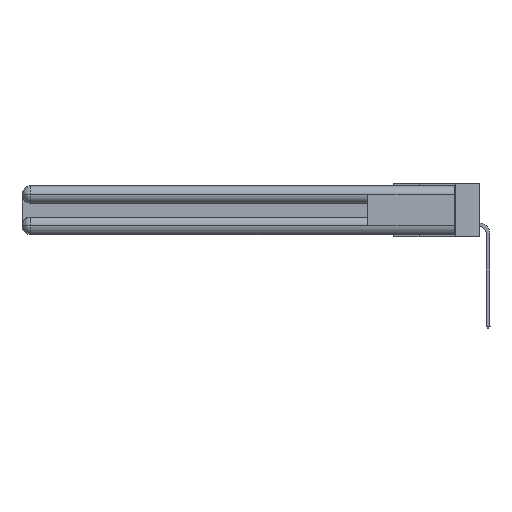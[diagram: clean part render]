
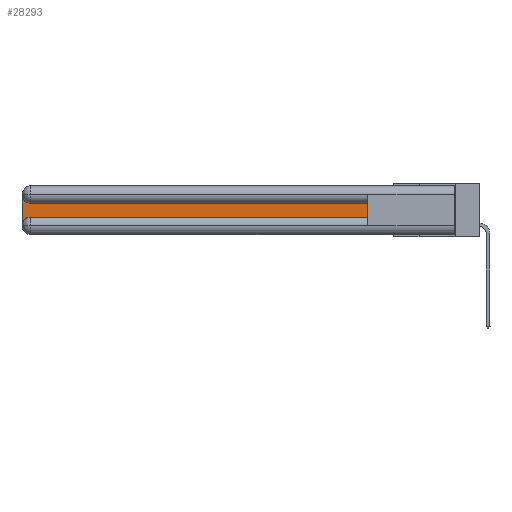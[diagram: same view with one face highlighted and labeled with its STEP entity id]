
A CAD part, left-side view. The second image highlights one B-rep face of the part: STEP entity #28293.
In plain terms, the highlighted planar face has unit normal (-1, 0, 0).
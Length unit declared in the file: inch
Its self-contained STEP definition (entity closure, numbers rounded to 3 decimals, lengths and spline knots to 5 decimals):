
#771 = VERTEX_POINT ( 'NONE', #12176 ) ;
#1724 = LINE ( 'NONE', #11737, #24600 ) ;
#2594 = ORIENTED_EDGE ( 'NONE', *, *, #15719, .T. ) ;
#4088 = DIRECTION ( 'NONE',  ( 1., 0., 0. ) ) ;
#4320 = CARTESIAN_POINT ( 'NONE',  ( 0.075, 3., -0.0625 ) ) ;
#4334 = VECTOR ( 'NONE', #18008, 39.37008 ) ;
#4375 = PLANE ( 'NONE',  #28291 ) ;
#5604 = VERTEX_POINT ( 'NONE', #19478 ) ;
#6372 = DIRECTION ( 'NONE',  ( 0., 0., -1. ) ) ;
#8468 = EDGE_CURVE ( 'NONE', #12946, #21386, #15218, .T. ) ;
#8684 = FACE_OUTER_BOUND ( 'NONE', #12983, .T. ) ;
#8936 = CARTESIAN_POINT ( 'NONE',  ( 0.075, 0.6, -0.1225 ) ) ;
#9541 = CARTESIAN_POINT ( 'NONE',  ( 0.075, 3., -0.1225 ) ) ;
#10247 = CARTESIAN_POINT ( 'NONE',  ( 0.075, 0.6, -0.2175 ) ) ;
#10462 = EDGE_CURVE ( 'NONE', #17507, #771, #27649, .T. ) ;
#11031 = CARTESIAN_POINT ( 'NONE',  ( 0.075, 2.94, -0.0625 ) ) ;
#11171 = ORIENTED_EDGE ( 'NONE', *, *, #8468, .T. ) ;
#11715 = CIRCLE ( 'NONE', #22199, 0.06 ) ;
#11737 = CARTESIAN_POINT ( 'NONE',  ( 0.075, 0.6, -0.2175 ) ) ;
#12176 = CARTESIAN_POINT ( 'NONE',  ( 0.075, 0.6, -0.2175 ) ) ;
#12946 = VERTEX_POINT ( 'NONE', #4320 ) ;
#12983 = EDGE_LOOP ( 'NONE', ( #19343, #2594, #11171, #23024, #16053, #21503 ) ) ;
#14130 = DIRECTION ( 'NONE',  ( 0., 0., 1. ) ) ;
#14459 = CARTESIAN_POINT ( 'NONE',  ( 0.075, 2.94, -0.2175 ) ) ;
#15218 = LINE ( 'NONE', #20277, #4334 ) ;
#15719 = EDGE_CURVE ( 'NONE', #5604, #12946, #28350, .T. ) ;
#16053 = ORIENTED_EDGE ( 'NONE', *, *, #10462, .T. ) ;
#16295 = EDGE_CURVE ( 'NONE', #771, #18937, #1724, .T. ) ;
#16494 = DIRECTION ( 'NONE',  ( 0., 1., 0. ) ) ;
#16663 = DIRECTION ( 'NONE',  ( 1., 0., 0. ) ) ;
#16953 = CARTESIAN_POINT ( 'NONE',  ( 0.075, 3., -0.2775 ) ) ;
#17507 = VERTEX_POINT ( 'NONE', #14459 ) ;
#18008 = DIRECTION ( 'NONE',  ( 0., 0., -1. ) ) ;
#18275 = VECTOR ( 'NONE', #16494, 39.37008 ) ;
#18671 = VECTOR ( 'NONE', #26953, 39.37008 ) ;
#18937 = VERTEX_POINT ( 'NONE', #8936 ) ;
#19009 = LINE ( 'NONE', #21049, #18275 ) ;
#19343 = ORIENTED_EDGE ( 'NONE', *, *, #25986, .T. ) ;
#19478 = CARTESIAN_POINT ( 'NONE',  ( 0.075, 2.94, -0.1225 ) ) ;
#19756 = DIRECTION ( 'NONE',  ( 0., 0., -1. ) ) ;
#20277 = CARTESIAN_POINT ( 'NONE',  ( 0.075, 3., -0.2175 ) ) ;
#21049 = CARTESIAN_POINT ( 'NONE',  ( 0.075, 0.6, -0.1225 ) ) ;
#21386 = VERTEX_POINT ( 'NONE', #16953 ) ;
#21503 = ORIENTED_EDGE ( 'NONE', *, *, #16295, .T. ) ;
#22199 = AXIS2_PLACEMENT_3D ( 'NONE', #27737, #25015, #19756 ) ;
#23024 = ORIENTED_EDGE ( 'NONE', *, *, #23595, .T. ) ;
#23551 = DIRECTION ( 'NONE',  ( 0., 0., -1. ) ) ;
#23595 = EDGE_CURVE ( 'NONE', #21386, #17507, #11715, .T. ) ;
#24600 = VECTOR ( 'NONE', #14130, 39.37008 ) ;
#25015 = DIRECTION ( 'NONE',  ( 1., 0., 0. ) ) ;
#25880 = AXIS2_PLACEMENT_3D ( 'NONE', #11031, #4088, #6372 ) ;
#25986 = EDGE_CURVE ( 'NONE', #18937, #5604, #19009, .T. ) ;
#26953 = DIRECTION ( 'NONE',  ( 0., -1., 0. ) ) ;
#27649 = LINE ( 'NONE', #10247, #18671 ) ;
#27737 = CARTESIAN_POINT ( 'NONE',  ( 0.075, 2.94, -0.2775 ) ) ;
#28291 = AXIS2_PLACEMENT_3D ( 'NONE', #9541, #16663, #23551 ) ;
#28293 = ADVANCED_FACE ( 'NONE', ( #8684 ), #4375, .F. ) ;
#28350 = CIRCLE ( 'NONE', #25880, 0.06 ) ;
